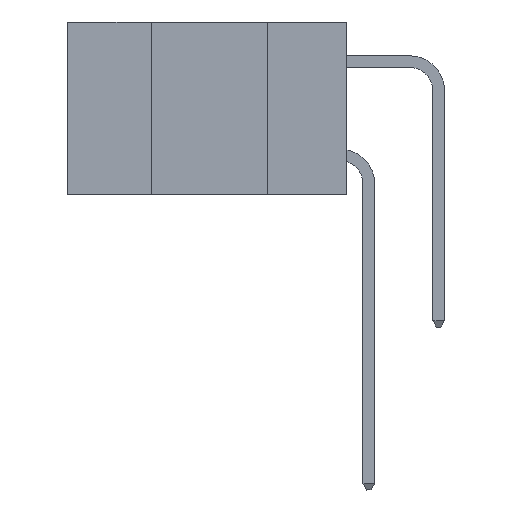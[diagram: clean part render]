
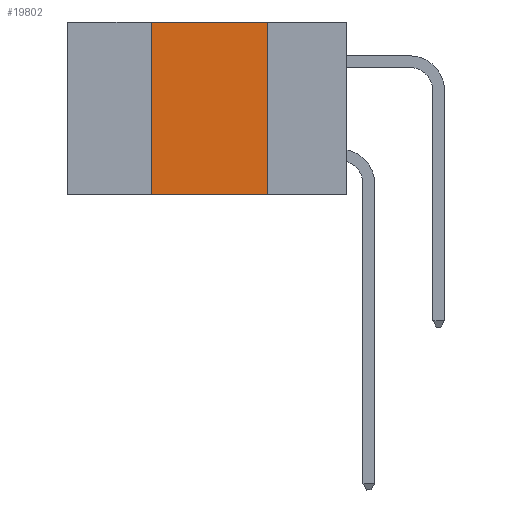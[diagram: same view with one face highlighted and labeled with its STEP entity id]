
A CAD part, left-side view. The second image highlights one B-rep face of the part: STEP entity #19802.
In plain terms, the highlighted planar face has unit normal (-1, 0, 0).
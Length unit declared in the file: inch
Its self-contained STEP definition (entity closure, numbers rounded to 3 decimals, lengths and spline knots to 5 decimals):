
#1199 = VERTEX_POINT ( 'NONE', #25172 ) ;
#1288 = CARTESIAN_POINT ( 'NONE',  ( 0., 0.17, -0.37 ) ) ;
#1737 = CARTESIAN_POINT ( 'NONE',  ( 0., 0.6, 0. ) ) ;
#2047 = DIRECTION ( 'NONE',  ( 0., 0., -1. ) ) ;
#2168 = PLANE ( 'NONE',  #10986 ) ;
#4339 = CARTESIAN_POINT ( 'NONE',  ( 0., 0.42, -0.37 ) ) ;
#4530 = LINE ( 'NONE', #25988, #18005 ) ;
#5353 = DIRECTION ( 'NONE',  ( 0., 0., 1. ) ) ;
#5886 = VERTEX_POINT ( 'NONE', #1288 ) ;
#7343 = LINE ( 'NONE', #15984, #21784 ) ;
#8259 = CARTESIAN_POINT ( 'NONE',  ( 0., 0.17, 0. ) ) ;
#8526 = FACE_OUTER_BOUND ( 'NONE', #18583, .T. ) ;
#9803 = VERTEX_POINT ( 'NONE', #4339 ) ;
#10127 = EDGE_CURVE ( 'NONE', #25837, #5886, #27717, .T. ) ;
#10666 = VECTOR ( 'NONE', #12922, 39.37008 ) ;
#10783 = DIRECTION ( 'NONE',  ( 0., 0., -1. ) ) ;
#10986 = AXIS2_PLACEMENT_3D ( 'NONE', #23706, #17589, #10783 ) ;
#11949 = EDGE_CURVE ( 'NONE', #1199, #25837, #19172, .T. ) ;
#12733 = ORIENTED_EDGE ( 'NONE', *, *, #10127, .F. ) ;
#12922 = DIRECTION ( 'NONE',  ( 0., -1., 0. ) ) ;
#13170 = DIRECTION ( 'NONE',  ( 0., -1., 0. ) ) ;
#14953 = ORIENTED_EDGE ( 'NONE', *, *, #26883, .T. ) ;
#15674 = EDGE_CURVE ( 'NONE', #9803, #1199, #7343, .T. ) ;
#15984 = CARTESIAN_POINT ( 'NONE',  ( 0., 0.42, 0. ) ) ;
#17589 = DIRECTION ( 'NONE',  ( 1., 0., 0. ) ) ;
#18005 = VECTOR ( 'NONE', #13170, 39.37008 ) ;
#18583 = EDGE_LOOP ( 'NONE', ( #12733, #22957, #27805, #14953 ) ) ;
#18790 = CARTESIAN_POINT ( 'NONE',  ( 0., 0.17, 0. ) ) ;
#19172 = LINE ( 'NONE', #1737, #10666 ) ;
#19802 = ADVANCED_FACE ( 'NONE', ( #8526 ), #2168, .F. ) ;
#21784 = VECTOR ( 'NONE', #5353, 39.37008 ) ;
#22957 = ORIENTED_EDGE ( 'NONE', *, *, #11949, .F. ) ;
#23571 = VECTOR ( 'NONE', #2047, 39.37008 ) ;
#23706 = CARTESIAN_POINT ( 'NONE',  ( 0., 0.6, 0. ) ) ;
#25172 = CARTESIAN_POINT ( 'NONE',  ( 0., 0.42, 0. ) ) ;
#25837 = VERTEX_POINT ( 'NONE', #18790 ) ;
#25988 = CARTESIAN_POINT ( 'NONE',  ( 0., 0.6, -0.37 ) ) ;
#26883 = EDGE_CURVE ( 'NONE', #9803, #5886, #4530, .T. ) ;
#27717 = LINE ( 'NONE', #8259, #23571 ) ;
#27805 = ORIENTED_EDGE ( 'NONE', *, *, #15674, .F. ) ;
